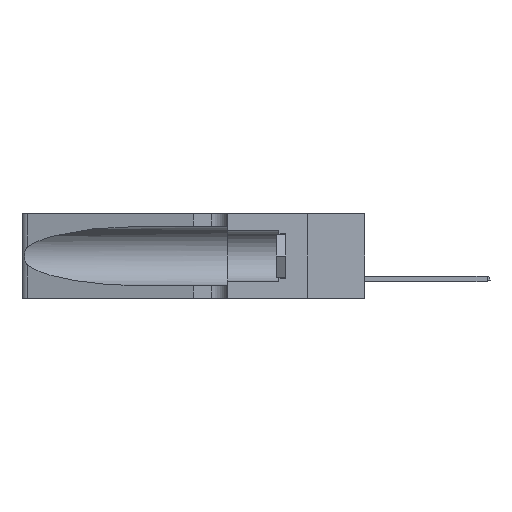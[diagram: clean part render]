
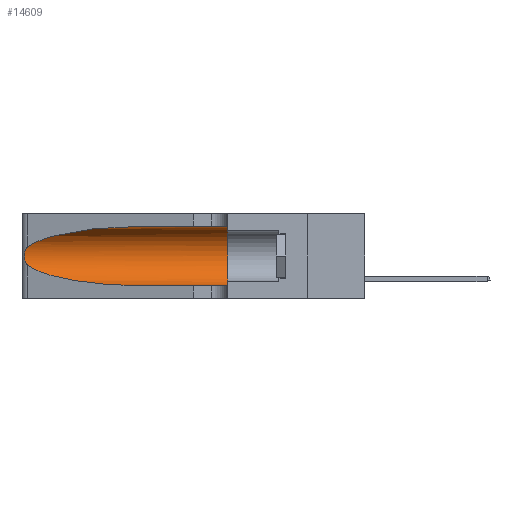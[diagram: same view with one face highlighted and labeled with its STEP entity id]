
A CAD part, left-side view. The second image highlights one B-rep face of the part: STEP entity #14609.
In plain terms, the highlighted cylindrical face has radius 3.308 mm (diameter 6.617 mm), a partial arc.
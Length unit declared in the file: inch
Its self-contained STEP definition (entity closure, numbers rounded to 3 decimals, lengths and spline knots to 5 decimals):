
#76 = CARTESIAN_POINT ( 'NONE',  ( 0.26075, 1.23896, 0.19203 ) ) ;
#80 = CARTESIAN_POINT ( 'NONE',  ( 0.1305, 0.72297, 0.05475 ) ) ;
#374 = CARTESIAN_POINT ( 'NONE',  ( 0.26018, 1.23835, 0.19895 ) ) ;
#463 = CARTESIAN_POINT ( 'NONE',  ( 0.2373, 1.15595, 0.28018 ) ) ;
#938 = ORIENTED_EDGE ( 'NONE', *, *, #12155, .F. ) ;
#1749 = ORIENTED_EDGE ( 'NONE', *, *, #2750, .T. ) ;
#2003 = CARTESIAN_POINT ( 'NONE',  ( 0.1305, 1.61858, 0.31525 ) ) ;
#2326 = CARTESIAN_POINT ( 'NONE',  ( 0.26075, 1.23896, 0.178 ) ) ;
#2511 = CARTESIAN_POINT ( 'NONE',  ( 0.25487, 1.22718, 0.14631 ) ) ;
#2750 = EDGE_CURVE ( 'NONE', #21023, #6941, #16565, .T. ) ;
#2987 = ORIENTED_EDGE ( 'NONE', *, *, #23154, .T. ) ;
#3707 =( BOUNDED_CURVE ( )  B_SPLINE_CURVE ( 3, ( #19675, #28620, #20243, #80 ),
 .UNSPECIFIED., .F., .F. ) 
 B_SPLINE_CURVE_WITH_KNOTS ( ( 4, 4 ),
 ( 3.44316, 4.71239 ),
 .UNSPECIFIED. ) 
 CURVE ( )  GEOMETRIC_REPRESENTATION_ITEM ( )  RATIONAL_B_SPLINE_CURVE ( ( 1., 0.87, 0.87, 1. ) ) 
 REPRESENTATION_ITEM ( '' )  );
#3746 = VERTEX_POINT ( 'NONE', #7657 ) ;
#3930 = CARTESIAN_POINT ( 'NONE',  ( 0.1305, 0.35, 0.185 ) ) ;
#4044 = VERTEX_POINT ( 'NONE', #8928 ) ;
#6342 = CARTESIAN_POINT ( 'NONE',  ( 0.1305, 1.61858, 0.05475 ) ) ;
#6505 = EDGE_CURVE ( 'NONE', #4044, #3746, #14459, .T. ) ;
#6941 = VERTEX_POINT ( 'NONE', #20669 ) ;
#7544 = CARTESIAN_POINT ( 'NONE',  ( 0.1305, 0.72297, 0.31525 ) ) ;
#7657 = CARTESIAN_POINT ( 'NONE',  ( 0.1305, 0.35, 0.05475 ) ) ;
#8431 = EDGE_CURVE ( 'NONE', #6941, #4044, #3707, .T. ) ;
#8856 = CARTESIAN_POINT ( 'NONE',  ( 0.25555, 1.22993, 0.14849 ) ) ;
#8928 = CARTESIAN_POINT ( 'NONE',  ( 0.1305, 0.72297, 0.05475 ) ) ;
#9653 = DIRECTION ( 'NONE',  ( 0., -1., 0. ) ) ;
#11015 = DIRECTION ( 'NONE',  ( 0., -1., 0. ) ) ;
#11289 = VERTEX_POINT ( 'NONE', #7544 ) ;
#11394 = CARTESIAN_POINT ( 'NONE',  ( 0.25789, 1.23486, 0.15765 ) ) ;
#11491 = CARTESIAN_POINT ( 'NONE',  ( 0.26017, 1.23833, 0.17102 ) ) ;
#12155 = EDGE_CURVE ( 'NONE', #28355, #3746, #13074, .T. ) ;
#12377 = CARTESIAN_POINT ( 'NONE',  ( 0.1305, 0.35, 0.31525 ) ) ;
#12523 = LINE ( 'NONE', #2003, #25074 ) ;
#12976 = DIRECTION ( 'NONE',  ( 0., 1., 0. ) ) ;
#13074 = CIRCLE ( 'NONE', #24875, 0.13025 ) ;
#13246 = DIRECTION ( 'NONE',  ( 0., 0., -1. ) ) ;
#14459 = LINE ( 'NONE', #6342, #24237 ) ;
#14609 = ADVANCED_FACE ( 'NONE', ( #14679 ), #18202, .F. ) ;
#14679 = FACE_OUTER_BOUND ( 'NONE', #21331, .T. ) ;
#14976 = CARTESIAN_POINT ( 'NONE',  ( 0.1305, 1.61858, 0.185 ) ) ;
#15081 = ORIENTED_EDGE ( 'NONE', *, *, #8431, .T. ) ;
#15756 = CARTESIAN_POINT ( 'NONE',  ( 0.1305, 0.72297, 0.31525 ) ) ;
#15761 = CARTESIAN_POINT ( 'NONE',  ( 0.25854, 1.2359, 0.20912 ) ) ;
#15805 = EDGE_CURVE ( 'NONE', #11289, #28355, #12523, .T. ) ;
#16213 =( BOUNDED_CURVE ( )  B_SPLINE_CURVE ( 3, ( #15756, #24725, #463, #25000 ),
 .UNSPECIFIED., .F., .F. ) 
 B_SPLINE_CURVE_WITH_KNOTS ( ( 4, 4 ),
 ( 1.5708, 2.84003 ),
 .UNSPECIFIED. ) 
 CURVE ( )  GEOMETRIC_REPRESENTATION_ITEM ( )  RATIONAL_B_SPLINE_CURVE ( ( 1., 0.87, 0.87, 1. ) ) 
 REPRESENTATION_ITEM ( '' )  );
#16565 = B_SPLINE_CURVE_WITH_KNOTS ( 'NONE', 3,
 ( #24816, #24633, #20041, #26867, #15761, #374, #76, #2326, #11491, #18106, #11394, #18010, #8856, #2511 ),
 .UNSPECIFIED., .F., .F.,
 ( 4, 2, 2, 2, 2, 2, 4 ),
 ( 0., 0.00027, 0.00053, 0.00107, 0.0016, 0.00187, 0.00214 ),
 .UNSPECIFIED. ) ;
#17838 = AXIS2_PLACEMENT_3D ( 'NONE', #14976, #11015, #13246 ) ;
#18010 = CARTESIAN_POINT ( 'NONE',  ( 0.25639, 1.23186, 0.15144 ) ) ;
#18106 = CARTESIAN_POINT ( 'NONE',  ( 0.25856, 1.23593, 0.16098 ) ) ;
#18202 = CYLINDRICAL_SURFACE ( 'NONE', #17838, 0.13025 ) ;
#19588 = ORIENTED_EDGE ( 'NONE', *, *, #6505, .T. ) ;
#19675 = CARTESIAN_POINT ( 'NONE',  ( 0.25487, 1.22718, 0.14631 ) ) ;
#20041 = CARTESIAN_POINT ( 'NONE',  ( 0.25639, 1.23184, 0.21858 ) ) ;
#20243 = CARTESIAN_POINT ( 'NONE',  ( 0.18966, 0.96281, 0.05475 ) ) ;
#20669 = CARTESIAN_POINT ( 'NONE',  ( 0.25487, 1.22718, 0.14631 ) ) ;
#21023 = VERTEX_POINT ( 'NONE', #28128 ) ;
#21302 = ORIENTED_EDGE ( 'NONE', *, *, #15805, .F. ) ;
#21331 = EDGE_LOOP ( 'NONE', ( #2987, #1749, #15081, #19588, #938, #21302 ) ) ;
#23154 = EDGE_CURVE ( 'NONE', #11289, #21023, #16213, .T. ) ;
#23959 = DIRECTION ( 'NONE',  ( 0., -1., 0. ) ) ;
#24237 = VECTOR ( 'NONE', #23959, 39.37008 ) ;
#24633 = CARTESIAN_POINT ( 'NONE',  ( 0.25555, 1.22994, 0.2215 ) ) ;
#24725 = CARTESIAN_POINT ( 'NONE',  ( 0.18966, 0.96281, 0.31525 ) ) ;
#24816 = CARTESIAN_POINT ( 'NONE',  ( 0.25487, 1.22718, 0.22369 ) ) ;
#24875 = AXIS2_PLACEMENT_3D ( 'NONE', #3930, #12976, #26405 ) ;
#25000 = CARTESIAN_POINT ( 'NONE',  ( 0.25487, 1.22718, 0.22369 ) ) ;
#25074 = VECTOR ( 'NONE', #9653, 39.37008 ) ;
#26405 = DIRECTION ( 'NONE',  ( 0., 0., 1. ) ) ;
#26867 = CARTESIAN_POINT ( 'NONE',  ( 0.25787, 1.23484, 0.2124 ) ) ;
#28128 = CARTESIAN_POINT ( 'NONE',  ( 0.25487, 1.22718, 0.22369 ) ) ;
#28355 = VERTEX_POINT ( 'NONE', #12377 ) ;
#28620 = CARTESIAN_POINT ( 'NONE',  ( 0.2373, 1.15595, 0.08982 ) ) ;
